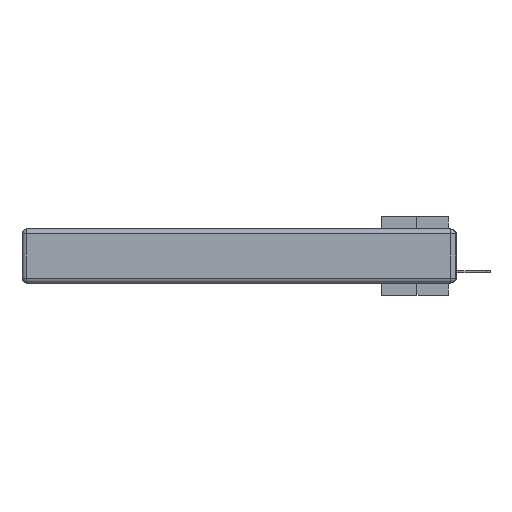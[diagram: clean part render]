
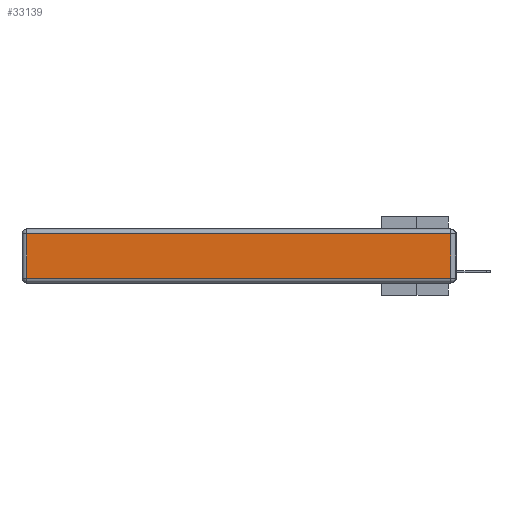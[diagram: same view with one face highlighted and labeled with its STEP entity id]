
A CAD part, left-side view. The second image highlights one B-rep face of the part: STEP entity #33139.
In plain terms, the highlighted planar face has unit normal (-1, 0, 0).
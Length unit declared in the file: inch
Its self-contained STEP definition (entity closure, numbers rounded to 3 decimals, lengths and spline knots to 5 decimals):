
#157 = VERTEX_POINT ( 'NONE', #14704 ) ;
#1118 = VERTEX_POINT ( 'NONE', #20926 ) ;
#1518 = EDGE_CURVE ( 'NONE', #157, #23535, #20230, .T. ) ;
#1520 = CARTESIAN_POINT ( 'NONE',  ( 0., 2.72, -0.343 ) ) ;
#2039 = FACE_OUTER_BOUND ( 'NONE', #21079, .T. ) ;
#3475 = ORIENTED_EDGE ( 'NONE', *, *, #27331, .T. ) ;
#4125 = CARTESIAN_POINT ( 'NONE',  ( 0., 2.72, -0.313 ) ) ;
#4699 = DIRECTION ( 'NONE',  ( 0., 0., 1. ) ) ;
#6400 = VECTOR ( 'NONE', #15762, 39.37008 ) ;
#6945 = AXIS2_PLACEMENT_3D ( 'NONE', #7734, #30998, #4699 ) ;
#7734 = CARTESIAN_POINT ( 'NONE',  ( 0., 0., -0.343 ) ) ;
#8401 = ORIENTED_EDGE ( 'NONE', *, *, #11163, .T. ) ;
#11163 = EDGE_CURVE ( 'NONE', #1118, #20615, #21758, .T. ) ;
#11760 = VECTOR ( 'NONE', #20535, 39.37008 ) ;
#13147 = CARTESIAN_POINT ( 'NONE',  ( 0., 0.03, -0.343 ) ) ;
#14207 = DIRECTION ( 'NONE',  ( 0., 0., -1. ) ) ;
#14704 = CARTESIAN_POINT ( 'NONE',  ( 0., 0.03, -0.313 ) ) ;
#15388 = CARTESIAN_POINT ( 'NONE',  ( 0., 0., -0.313 ) ) ;
#15762 = DIRECTION ( 'NONE',  ( 0., 0., 1. ) ) ;
#15971 = ORIENTED_EDGE ( 'NONE', *, *, #1518, .T. ) ;
#16184 = LINE ( 'NONE', #15388, #11760 ) ;
#16469 = CARTESIAN_POINT ( 'NONE',  ( 0., 0.03, -0.03 ) ) ;
#17693 = CARTESIAN_POINT ( 'NONE',  ( 0., 2.75, -0.03 ) ) ;
#20077 = ORIENTED_EDGE ( 'NONE', *, *, #27548, .T. ) ;
#20230 = LINE ( 'NONE', #13147, #6400 ) ;
#20535 = DIRECTION ( 'NONE',  ( 0., -1., 0. ) ) ;
#20615 = VERTEX_POINT ( 'NONE', #4125 ) ;
#20704 = VECTOR ( 'NONE', #33338, 39.37008 ) ;
#20926 = CARTESIAN_POINT ( 'NONE',  ( 0., 2.72, -0.03 ) ) ;
#21079 = EDGE_LOOP ( 'NONE', ( #20077, #15971, #3475, #8401 ) ) ;
#21758 = LINE ( 'NONE', #1520, #25401 ) ;
#23535 = VERTEX_POINT ( 'NONE', #16469 ) ;
#25401 = VECTOR ( 'NONE', #14207, 39.37008 ) ;
#27331 = EDGE_CURVE ( 'NONE', #23535, #1118, #32874, .T. ) ;
#27548 = EDGE_CURVE ( 'NONE', #20615, #157, #16184, .T. ) ;
#28276 = PLANE ( 'NONE',  #6945 ) ;
#30998 = DIRECTION ( 'NONE',  ( -1., 0., 0. ) ) ;
#32874 = LINE ( 'NONE', #17693, #20704 ) ;
#33139 = ADVANCED_FACE ( 'NONE', ( #2039 ), #28276, .T. ) ;
#33338 = DIRECTION ( 'NONE',  ( 0., 1., 0. ) ) ;
